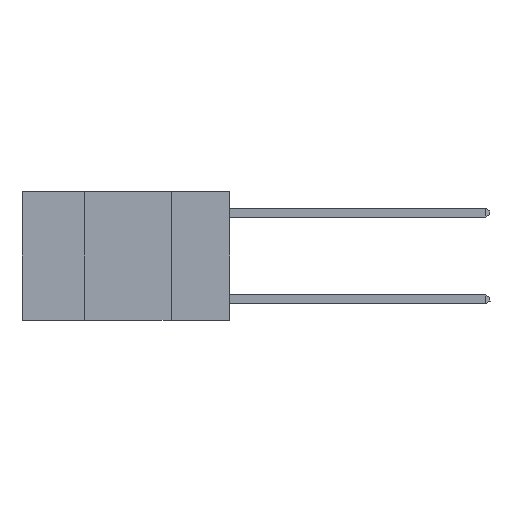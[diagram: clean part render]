
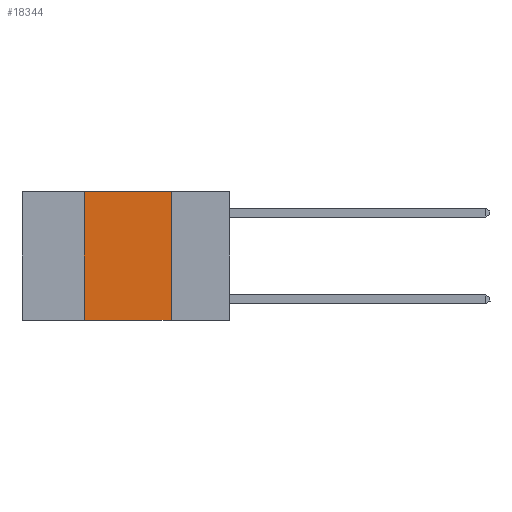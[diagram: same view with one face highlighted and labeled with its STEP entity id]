
A CAD part, left-side view. The second image highlights one B-rep face of the part: STEP entity #18344.
In plain terms, the highlighted planar face has unit normal (-1, 0, 0).
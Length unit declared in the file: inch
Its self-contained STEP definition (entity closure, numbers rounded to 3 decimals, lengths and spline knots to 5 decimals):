
#267 = CARTESIAN_POINT ( 'NONE',  ( 0., 0.6, 0. ) ) ;
#2289 = EDGE_CURVE ( 'NONE', #13412, #17970, #16125, .T. ) ;
#3076 = EDGE_CURVE ( 'NONE', #13412, #19444, #27319, .T. ) ;
#3939 = CARTESIAN_POINT ( 'NONE',  ( 0., 0.17, -0.37 ) ) ;
#4244 = VECTOR ( 'NONE', #5942, 39.37008 ) ;
#4340 = DIRECTION ( 'NONE',  ( 0., 0., 1. ) ) ;
#4956 = LINE ( 'NONE', #267, #16826 ) ;
#5885 = CARTESIAN_POINT ( 'NONE',  ( 0., 0.42, -0.37 ) ) ;
#5942 = DIRECTION ( 'NONE',  ( 0., -1., 0. ) ) ;
#5988 = CARTESIAN_POINT ( 'NONE',  ( 0., 0.42, 0. ) ) ;
#6083 = EDGE_CURVE ( 'NONE', #7168, #17970, #7593, .T. ) ;
#7168 = VERTEX_POINT ( 'NONE', #23369 ) ;
#7280 = PLANE ( 'NONE',  #7609 ) ;
#7593 = LINE ( 'NONE', #17863, #19397 ) ;
#7609 = AXIS2_PLACEMENT_3D ( 'NONE', #22739, #11739, #27075 ) ;
#8263 = EDGE_CURVE ( 'NONE', #19444, #7168, #4956, .T. ) ;
#9797 = VECTOR ( 'NONE', #4340, 39.37008 ) ;
#11739 = DIRECTION ( 'NONE',  ( 1., 0., 0. ) ) ;
#12405 = ORIENTED_EDGE ( 'NONE', *, *, #6083, .F. ) ;
#12669 = CARTESIAN_POINT ( 'NONE',  ( 0., 0.6, -0.37 ) ) ;
#13111 = ORIENTED_EDGE ( 'NONE', *, *, #8263, .F. ) ;
#13412 = VERTEX_POINT ( 'NONE', #5885 ) ;
#14452 = EDGE_LOOP ( 'NONE', ( #12405, #13111, #25469, #21360 ) ) ;
#15464 = CARTESIAN_POINT ( 'NONE',  ( 0., 0.42, 0. ) ) ;
#15930 = DIRECTION ( 'NONE',  ( 0., -1., 0. ) ) ;
#16125 = LINE ( 'NONE', #12669, #4244 ) ;
#16826 = VECTOR ( 'NONE', #15930, 39.37008 ) ;
#17863 = CARTESIAN_POINT ( 'NONE',  ( 0., 0.17, 0. ) ) ;
#17970 = VERTEX_POINT ( 'NONE', #3939 ) ;
#18344 = ADVANCED_FACE ( 'NONE', ( #22126 ), #7280, .F. ) ;
#19397 = VECTOR ( 'NONE', #20075, 39.37008 ) ;
#19444 = VERTEX_POINT ( 'NONE', #5988 ) ;
#20075 = DIRECTION ( 'NONE',  ( 0., 0., -1. ) ) ;
#21360 = ORIENTED_EDGE ( 'NONE', *, *, #2289, .T. ) ;
#22126 = FACE_OUTER_BOUND ( 'NONE', #14452, .T. ) ;
#22739 = CARTESIAN_POINT ( 'NONE',  ( 0., 0.6, 0. ) ) ;
#23369 = CARTESIAN_POINT ( 'NONE',  ( 0., 0.17, 0. ) ) ;
#25469 = ORIENTED_EDGE ( 'NONE', *, *, #3076, .F. ) ;
#27075 = DIRECTION ( 'NONE',  ( 0., 0., -1. ) ) ;
#27319 = LINE ( 'NONE', #15464, #9797 ) ;
